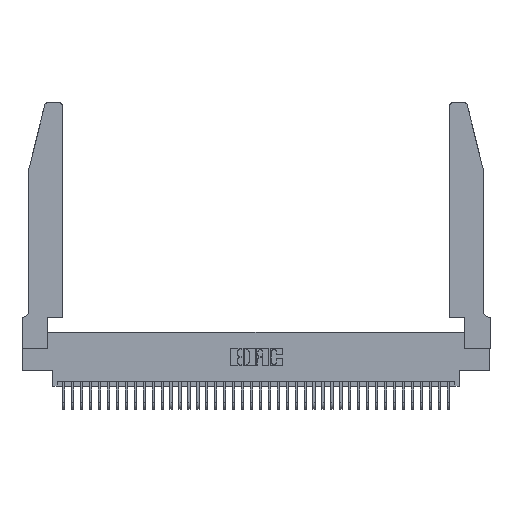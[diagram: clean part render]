
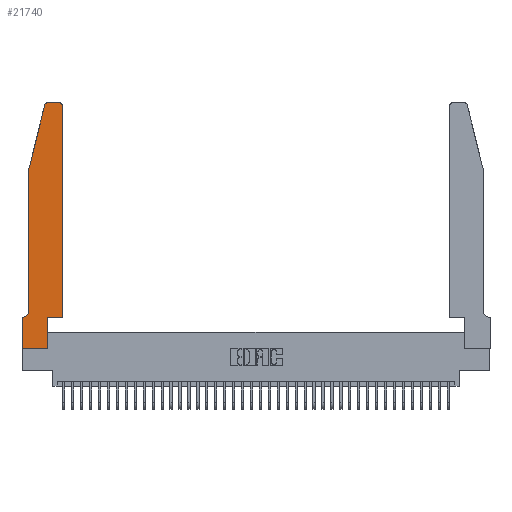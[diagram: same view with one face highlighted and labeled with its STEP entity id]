
A CAD part, top view. The second image highlights one B-rep face of the part: STEP entity #21740.
In plain terms, the highlighted planar face has unit normal (0, 0, 1).
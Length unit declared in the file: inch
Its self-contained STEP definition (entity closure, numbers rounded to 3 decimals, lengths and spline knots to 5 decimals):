
#443 = AXIS2_PLACEMENT_3D ( 'NONE', #21584, #9019, #21309 ) ;
#710 = DIRECTION ( 'NONE',  ( 1., 0., 0. ) ) ;
#935 = DIRECTION ( 'NONE',  ( 0., 1., 0. ) ) ;
#1322 = DIRECTION ( 'NONE',  ( -0.239, -0.971, 0. ) ) ;
#1643 = VERTEX_POINT ( 'NONE', #16169 ) ;
#2673 = DIRECTION ( 'NONE',  ( 1., 0., 0. ) ) ;
#3378 = VECTOR ( 'NONE', #2673, 39.37008 ) ;
#3478 = CARTESIAN_POINT ( 'NONE',  ( 0., 0., 0.37 ) ) ;
#3700 = VERTEX_POINT ( 'NONE', #6390 ) ;
#3990 = ORIENTED_EDGE ( 'NONE', *, *, #12170, .T. ) ;
#4042 = CIRCLE ( 'NONE', #21822, 0.03 ) ;
#4646 = ORIENTED_EDGE ( 'NONE', *, *, #7024, .T. ) ;
#4794 = EDGE_LOOP ( 'NONE', ( #33872, #33138, #5117, #15979, #19675, #33222, #23342, #3990, #4646, #34715, #26686, #16355 ) ) ;
#5117 = ORIENTED_EDGE ( 'NONE', *, *, #20484, .T. ) ;
#5137 = VECTOR ( 'NONE', #20372, 39.37008 ) ;
#5415 = VERTEX_POINT ( 'NONE', #22459 ) ;
#5451 = CARTESIAN_POINT ( 'NONE',  ( 0.0755, 0.42, 0.37 ) ) ;
#5805 = AXIS2_PLACEMENT_3D ( 'NONE', #16011, #13246, #710 ) ;
#6390 = CARTESIAN_POINT ( 'NONE',  ( 0.25487, 2.72718, 0.37 ) ) ;
#7024 = EDGE_CURVE ( 'NONE', #5415, #32781, #39263, .T. ) ;
#7866 = VERTEX_POINT ( 'NONE', #5451 ) ;
#7880 = VECTOR ( 'NONE', #1322, 39.37008 ) ;
#7889 = DIRECTION ( 'NONE',  ( 1., 0., 0. ) ) ;
#8211 = CARTESIAN_POINT ( 'NONE',  ( 0., 0., 0.37 ) ) ;
#9019 = DIRECTION ( 'NONE',  ( 0., 0., -1. ) ) ;
#9971 = EDGE_CURVE ( 'NONE', #39956, #15452, #4042, .T. ) ;
#10060 = VERTEX_POINT ( 'NONE', #20575 ) ;
#10762 = FACE_OUTER_BOUND ( 'NONE', #4794, .T. ) ;
#10979 = EDGE_CURVE ( 'NONE', #36072, #31834, #37502, .T. ) ;
#12170 = EDGE_CURVE ( 'NONE', #31834, #5415, #18163, .T. ) ;
#12754 = CARTESIAN_POINT ( 'NONE',  ( 0.2605, 2.75, 0.37 ) ) ;
#13246 = DIRECTION ( 'NONE',  ( 0., 0., 1. ) ) ;
#14371 = EDGE_CURVE ( 'NONE', #34542, #3700, #22338, .T. ) ;
#14462 = LINE ( 'NONE', #33399, #36182 ) ;
#14805 = LINE ( 'NONE', #36047, #7880 ) ;
#15452 = VERTEX_POINT ( 'NONE', #23592 ) ;
#15979 = ORIENTED_EDGE ( 'NONE', *, *, #19919, .T. ) ;
#16011 = CARTESIAN_POINT ( 'NONE',  ( 0.284, 2.72, 0.37 ) ) ;
#16169 = CARTESIAN_POINT ( 'NONE',  ( 0.4505, 0.35, 0.37 ) ) ;
#16355 = ORIENTED_EDGE ( 'NONE', *, *, #9971, .T. ) ;
#17290 = VECTOR ( 'NONE', #28136, 39.37008 ) ;
#17894 = CARTESIAN_POINT ( 'NONE',  ( 0.2865, 0.35, 0.37 ) ) ;
#18163 = LINE ( 'NONE', #8211, #3378 ) ;
#18468 = VECTOR ( 'NONE', #935, 39.37008 ) ;
#19020 = CARTESIAN_POINT ( 'NONE',  ( 0.0055, 0.35, 0.37 ) ) ;
#19418 = CARTESIAN_POINT ( 'NONE',  ( 0.4505, 2.72, 0.37 ) ) ;
#19675 = ORIENTED_EDGE ( 'NONE', *, *, #33530, .T. ) ;
#19729 = VECTOR ( 'NONE', #25157, 39.37008 ) ;
#19919 = EDGE_CURVE ( 'NONE', #10060, #7866, #21937, .T. ) ;
#19945 = LINE ( 'NONE', #26137, #18468 ) ;
#20212 = DIRECTION ( 'NONE',  ( 0., 1., 0. ) ) ;
#20372 = DIRECTION ( 'NONE',  ( 0., -1., 0. ) ) ;
#20484 = EDGE_CURVE ( 'NONE', #3700, #10060, #14805, .T. ) ;
#20575 = CARTESIAN_POINT ( 'NONE',  ( 0.0755, 2., 0.37 ) ) ;
#21138 = EDGE_CURVE ( 'NONE', #15452, #34542, #36486, .T. ) ;
#21309 = DIRECTION ( 'NONE',  ( -1., 0., 0. ) ) ;
#21584 = CARTESIAN_POINT ( 'NONE',  ( 0.0055, 0.42, 0.37 ) ) ;
#21740 = ADVANCED_FACE ( 'NONE', ( #10762 ), #34077, .T. ) ;
#21822 = AXIS2_PLACEMENT_3D ( 'NONE', #33275, #36562, #7889 ) ;
#21937 = LINE ( 'NONE', #39546, #5137 ) ;
#22104 = DIRECTION ( 'NONE',  ( 1., 0., 0. ) ) ;
#22338 = CIRCLE ( 'NONE', #5805, 0.03 ) ;
#22459 = CARTESIAN_POINT ( 'NONE',  ( 0.2865, 0., 0.37 ) ) ;
#23342 = ORIENTED_EDGE ( 'NONE', *, *, #10979, .T. ) ;
#23404 = CARTESIAN_POINT ( 'NONE',  ( 0.284, 2.75, 0.37 ) ) ;
#23592 = CARTESIAN_POINT ( 'NONE',  ( 0.4205, 2.75, 0.37 ) ) ;
#24682 = CARTESIAN_POINT ( 'NONE',  ( 0., 0.35, 0.37 ) ) ;
#25011 = EDGE_CURVE ( 'NONE', #32781, #1643, #14462, .T. ) ;
#25138 = CARTESIAN_POINT ( 'NONE',  ( 0., 0.35, 0.37 ) ) ;
#25157 = DIRECTION ( 'NONE',  ( -1., 0., 0. ) ) ;
#25549 = AXIS2_PLACEMENT_3D ( 'NONE', #24682, #37247, #22104 ) ;
#26137 = CARTESIAN_POINT ( 'NONE',  ( 0.4505, 0.35, 0.37 ) ) ;
#26686 = ORIENTED_EDGE ( 'NONE', *, *, #27455, .T. ) ;
#27010 = DIRECTION ( 'NONE',  ( -1., 0., 0. ) ) ;
#27455 = EDGE_CURVE ( 'NONE', #1643, #39956, #19945, .T. ) ;
#28136 = DIRECTION ( 'NONE',  ( 0., -1., 0. ) ) ;
#28261 = EDGE_CURVE ( 'NONE', #28480, #36072, #36622, .T. ) ;
#28480 = VERTEX_POINT ( 'NONE', #19020 ) ;
#29971 = CARTESIAN_POINT ( 'NONE',  ( 0., 0., 0.37 ) ) ;
#30645 = DIRECTION ( 'NONE',  ( 1., 0., 0. ) ) ;
#31834 = VERTEX_POINT ( 'NONE', #3478 ) ;
#32781 = VERTEX_POINT ( 'NONE', #17894 ) ;
#32934 = CARTESIAN_POINT ( 'NONE',  ( 0.2865, 0.35, 0.37 ) ) ;
#33138 = ORIENTED_EDGE ( 'NONE', *, *, #14371, .T. ) ;
#33222 = ORIENTED_EDGE ( 'NONE', *, *, #28261, .T. ) ;
#33275 = CARTESIAN_POINT ( 'NONE',  ( 0.4205, 2.72, 0.37 ) ) ;
#33399 = CARTESIAN_POINT ( 'NONE',  ( 0.4505, 0.35, 0.37 ) ) ;
#33530 = EDGE_CURVE ( 'NONE', #7866, #28480, #34016, .T. ) ;
#33872 = ORIENTED_EDGE ( 'NONE', *, *, #21138, .T. ) ;
#34016 = CIRCLE ( 'NONE', #443, 0.07 ) ;
#34077 = PLANE ( 'NONE',  #25549 ) ;
#34542 = VERTEX_POINT ( 'NONE', #23404 ) ;
#34715 = ORIENTED_EDGE ( 'NONE', *, *, #25011, .T. ) ;
#36047 = CARTESIAN_POINT ( 'NONE',  ( 0.0755, 2., 0.37 ) ) ;
#36072 = VERTEX_POINT ( 'NONE', #25138 ) ;
#36182 = VECTOR ( 'NONE', #30645, 39.37008 ) ;
#36486 = LINE ( 'NONE', #12754, #19729 ) ;
#36562 = DIRECTION ( 'NONE',  ( 0., 0., 1. ) ) ;
#36622 = LINE ( 'NONE', #39971, #40056 ) ;
#37247 = DIRECTION ( 'NONE',  ( 0., 0., 1. ) ) ;
#37502 = LINE ( 'NONE', #29971, #17290 ) ;
#37797 = VECTOR ( 'NONE', #20212, 39.37008 ) ;
#39263 = LINE ( 'NONE', #32934, #37797 ) ;
#39546 = CARTESIAN_POINT ( 'NONE',  ( 0.0755, 2., 0.37 ) ) ;
#39956 = VERTEX_POINT ( 'NONE', #19418 ) ;
#39971 = CARTESIAN_POINT ( 'NONE',  ( 0.0755, 0.35, 0.37 ) ) ;
#40056 = VECTOR ( 'NONE', #27010, 39.37008 ) ;
